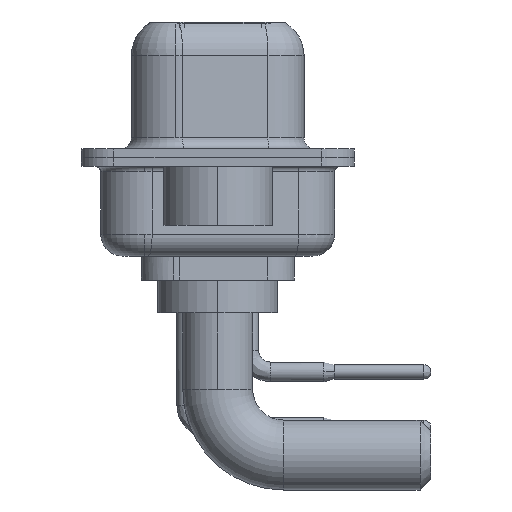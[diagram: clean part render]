
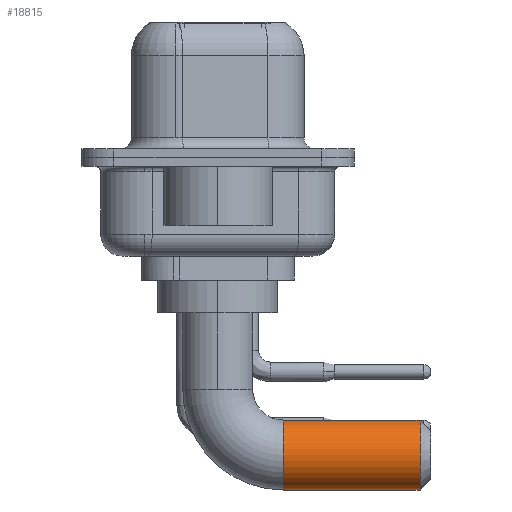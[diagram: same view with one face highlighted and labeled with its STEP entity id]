
A CAD part, left-side view. The second image highlights one B-rep face of the part: STEP entity #18815.
In plain terms, the highlighted cylindrical face has radius 1.6 mm (diameter 3.2 mm), a partial arc.
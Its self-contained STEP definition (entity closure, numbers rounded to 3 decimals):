
#341 = ORIENTED_EDGE ( 'NONE', *, *, #5635, .T. ) ;
#452 = VERTEX_POINT ( 'NONE', #12290 ) ;
#592 = VERTEX_POINT ( 'NONE', #18524 ) ;
#1691 = DIRECTION ( 'NONE',  ( 0., 1., 0. ) ) ;
#2208 = AXIS2_PLACEMENT_3D ( 'NONE', #12878, #1691, #20327 ) ;
#4117 = CARTESIAN_POINT ( 'NONE',  ( 0., -9.25, -4.9 ) ) ;
#4347 = CARTESIAN_POINT ( 'NONE',  ( 0., -3., -6.5 ) ) ;
#5635 = EDGE_CURVE ( 'NONE', #15044, #18053, #14488, .T. ) ;
#5759 = ORIENTED_EDGE ( 'NONE', *, *, #18059, .T. ) ;
#6690 = CIRCLE ( 'NONE', #21664, 1.6 ) ;
#7658 = CYLINDRICAL_SURFACE ( 'NONE', #11742, 1.6 ) ;
#7776 = FACE_OUTER_BOUND ( 'NONE', #15138, .T. ) ;
#8023 = LINE ( 'NONE', #9598, #20065 ) ;
#8548 = CARTESIAN_POINT ( 'NONE',  ( 0., -3., -8.1 ) ) ;
#9231 = DIRECTION ( 'NONE',  ( 0., -1., 0. ) ) ;
#9598 = CARTESIAN_POINT ( 'NONE',  ( 0., -3., -4.9 ) ) ;
#9995 = LINE ( 'NONE', #8548, #10152 ) ;
#10117 = DIRECTION ( 'NONE',  ( 0., -1., 0. ) ) ;
#10152 = VECTOR ( 'NONE', #10117, 1000. ) ;
#11742 = AXIS2_PLACEMENT_3D ( 'NONE', #22323, #9231, #16900 ) ;
#12290 = CARTESIAN_POINT ( 'NONE',  ( 0., -3., -4.9 ) ) ;
#12878 = CARTESIAN_POINT ( 'NONE',  ( 0., -9.25, -6.5 ) ) ;
#13920 = ORIENTED_EDGE ( 'NONE', *, *, #17890, .T. ) ;
#14488 = CIRCLE ( 'NONE', #2208, 1.6 ) ;
#14790 = EDGE_CURVE ( 'NONE', #452, #18053, #8023, .T. ) ;
#15044 = VERTEX_POINT ( 'NONE', #18050 ) ;
#15138 = EDGE_LOOP ( 'NONE', ( #21532, #13920, #5759, #341 ) ) ;
#16900 = DIRECTION ( 'NONE',  ( 0., 0., -1. ) ) ;
#17890 = EDGE_CURVE ( 'NONE', #452, #592, #6690, .T. ) ;
#18050 = CARTESIAN_POINT ( 'NONE',  ( 0., -9.25, -8.1 ) ) ;
#18053 = VERTEX_POINT ( 'NONE', #4117 ) ;
#18059 = EDGE_CURVE ( 'NONE', #592, #15044, #9995, .T. ) ;
#18331 = DIRECTION ( 'NONE',  ( -1., 0., 0. ) ) ;
#18524 = CARTESIAN_POINT ( 'NONE',  ( 0., -3., -8.1 ) ) ;
#18768 = DIRECTION ( 'NONE',  ( 0., -1., 0. ) ) ;
#18815 = ADVANCED_FACE ( 'NONE', ( #7776 ), #7658, .T. ) ;
#20065 = VECTOR ( 'NONE', #20892, 1000. ) ;
#20327 = DIRECTION ( 'NONE',  ( 0., 0., -1. ) ) ;
#20892 = DIRECTION ( 'NONE',  ( 0., -1., 0. ) ) ;
#21532 = ORIENTED_EDGE ( 'NONE', *, *, #14790, .F. ) ;
#21664 = AXIS2_PLACEMENT_3D ( 'NONE', #4347, #18768, #18331 ) ;
#22323 = CARTESIAN_POINT ( 'NONE',  ( 0., -3., -6.5 ) ) ;
